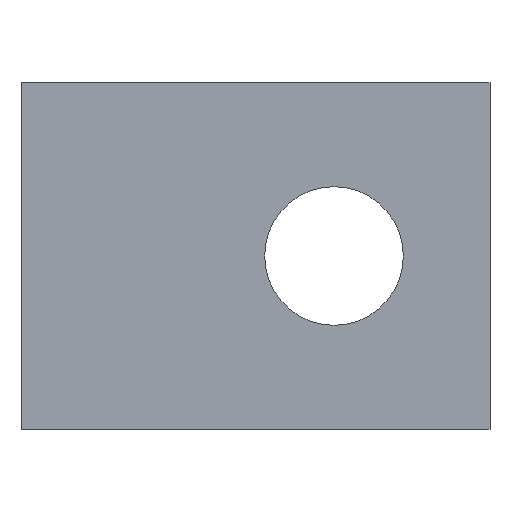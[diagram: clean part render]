
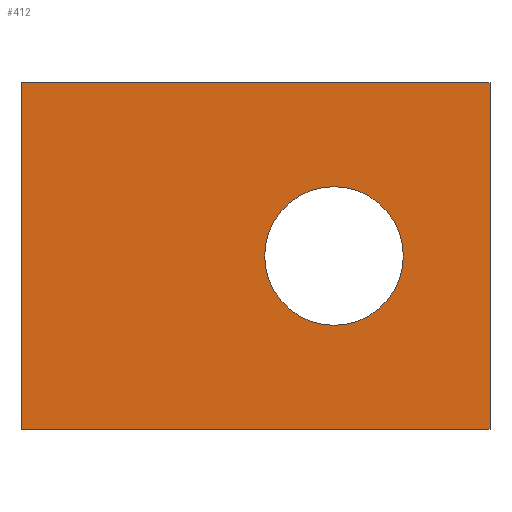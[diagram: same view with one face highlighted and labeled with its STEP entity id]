
A CAD part, front view. The second image highlights one B-rep face of the part: STEP entity #412.
In plain terms, the highlighted planar face has unit normal (0, -1, 0).
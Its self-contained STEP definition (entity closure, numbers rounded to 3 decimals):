
#9 = AXIS2_PLACEMENT_3D ( 'NONE', #485, #45, #289 ) ;
#28 = CARTESIAN_POINT ( 'NONE',  ( -14.337, -7.414, 0. ) ) ;
#31 = VERTEX_POINT ( 'NONE', #476 ) ;
#40 = DIRECTION ( 'NONE',  ( 1., 0., 0. ) ) ;
#45 = DIRECTION ( 'NONE',  ( 0., 1., 0. ) ) ;
#48 = CARTESIAN_POINT ( 'NONE',  ( -25.337, -7.414, -5. ) ) ;
#57 = ORIENTED_EDGE ( 'NONE', *, *, #304, .T. ) ;
#76 = EDGE_LOOP ( 'NONE', ( #632, #573, #467, #57 ) ) ;
#85 = VERTEX_POINT ( 'NONE', #422 ) ;
#107 = DIRECTION ( 'NONE',  ( 0., 1., 0. ) ) ;
#116 = VECTOR ( 'NONE', #559, 1000. ) ;
#120 = DIRECTION ( 'NONE',  ( -1., 0., 0. ) ) ;
#143 = LINE ( 'NONE', #503, #508 ) ;
#159 = VERTEX_POINT ( 'NONE', #646 ) ;
#204 = VECTOR ( 'NONE', #120, 1000. ) ;
#206 = DIRECTION ( 'NONE',  ( 1., 0., 0. ) ) ;
#211 = EDGE_CURVE ( 'NONE', #31, #393, #619, .T. ) ;
#216 = CARTESIAN_POINT ( 'NONE',  ( -11.837, -7.414, -5. ) ) ;
#247 = CARTESIAN_POINT ( 'NONE',  ( -25.337, -7.414, -5. ) ) ;
#261 = CIRCLE ( 'NONE', #9, 2. ) ;
#278 = EDGE_CURVE ( 'NONE', #617, #617, #261, .T. ) ;
#282 = AXIS2_PLACEMENT_3D ( 'NONE', #48, #107, #206 ) ;
#289 = DIRECTION ( 'NONE',  ( 1., 0., 0. ) ) ;
#300 = EDGE_CURVE ( 'NONE', #159, #85, #409, .T. ) ;
#304 = EDGE_CURVE ( 'NONE', #85, #31, #143, .T. ) ;
#337 = EDGE_CURVE ( 'NONE', #393, #159, #392, .T. ) ;
#340 = VECTOR ( 'NONE', #40, 1000. ) ;
#392 = LINE ( 'NONE', #216, #116 ) ;
#393 = VERTEX_POINT ( 'NONE', #397 ) ;
#397 = CARTESIAN_POINT ( 'NONE',  ( -11.837, -7.414, -5. ) ) ;
#399 = FACE_BOUND ( 'NONE', #517, .T. ) ;
#409 = LINE ( 'NONE', #440, #204 ) ;
#412 = ADVANCED_FACE ( 'NONE', ( #565, #399 ), #549, .F. ) ;
#422 = CARTESIAN_POINT ( 'NONE',  ( -25.337, -7.414, 5. ) ) ;
#440 = CARTESIAN_POINT ( 'NONE',  ( -11.837, -7.414, 5. ) ) ;
#455 = DIRECTION ( 'NONE',  ( 0., 0., -1. ) ) ;
#467 = ORIENTED_EDGE ( 'NONE', *, *, #300, .T. ) ;
#476 = CARTESIAN_POINT ( 'NONE',  ( -25.337, -7.414, -5. ) ) ;
#485 = CARTESIAN_POINT ( 'NONE',  ( -16.337, -7.414, 0. ) ) ;
#503 = CARTESIAN_POINT ( 'NONE',  ( -25.337, -7.414, 5. ) ) ;
#508 = VECTOR ( 'NONE', #455, 1000. ) ;
#517 = EDGE_LOOP ( 'NONE', ( #624 ) ) ;
#549 = PLANE ( 'NONE',  #282 ) ;
#559 = DIRECTION ( 'NONE',  ( 0., 0., 1. ) ) ;
#565 = FACE_OUTER_BOUND ( 'NONE', #76, .T. ) ;
#573 = ORIENTED_EDGE ( 'NONE', *, *, #337, .T. ) ;
#617 = VERTEX_POINT ( 'NONE', #28 ) ;
#619 = LINE ( 'NONE', #247, #340 ) ;
#624 = ORIENTED_EDGE ( 'NONE', *, *, #278, .T. ) ;
#632 = ORIENTED_EDGE ( 'NONE', *, *, #211, .T. ) ;
#646 = CARTESIAN_POINT ( 'NONE',  ( -11.837, -7.414, 5. ) ) ;
